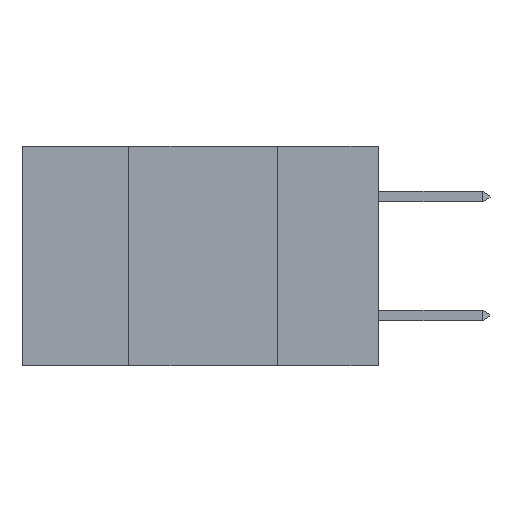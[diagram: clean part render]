
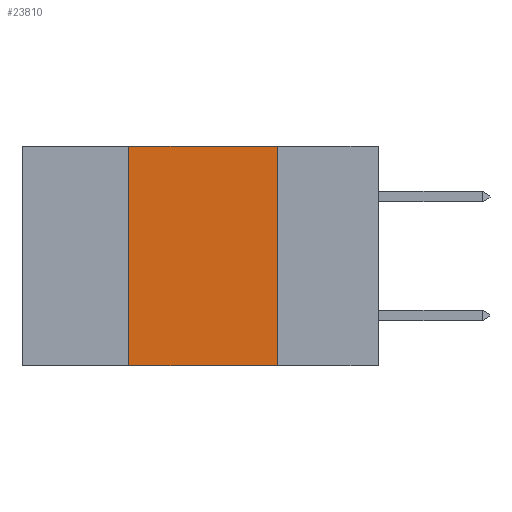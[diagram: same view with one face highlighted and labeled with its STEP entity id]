
A CAD part, left-side view. The second image highlights one B-rep face of the part: STEP entity #23810.
In plain terms, the highlighted planar face has unit normal (-1, 0, 0).
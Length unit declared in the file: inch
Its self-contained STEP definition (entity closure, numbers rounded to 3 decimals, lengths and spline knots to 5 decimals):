
#180 = DIRECTION ( 'NONE',  ( 0., 0., 1. ) ) ;
#444 = ORIENTED_EDGE ( 'NONE', *, *, #26952, .F. ) ;
#778 = VECTOR ( 'NONE', #26306, 39.37008 ) ;
#2094 = FACE_OUTER_BOUND ( 'NONE', #16091, .T. ) ;
#2271 = CARTESIAN_POINT ( 'NONE',  ( 0., 0.42, -0.37 ) ) ;
#2876 = VECTOR ( 'NONE', #19764, 39.37008 ) ;
#3628 = AXIS2_PLACEMENT_3D ( 'NONE', #6539, #8759, #23642 ) ;
#4465 = PLANE ( 'NONE',  #3628 ) ;
#6539 = CARTESIAN_POINT ( 'NONE',  ( 0., 0.6, 0. ) ) ;
#7000 = CARTESIAN_POINT ( 'NONE',  ( 0., 0.6, -0.37 ) ) ;
#8008 = LINE ( 'NONE', #15109, #14369 ) ;
#8246 = EDGE_CURVE ( 'NONE', #8930, #19186, #8008, .T. ) ;
#8759 = DIRECTION ( 'NONE',  ( 1., 0., 0. ) ) ;
#8930 = VERTEX_POINT ( 'NONE', #2271 ) ;
#9194 = CARTESIAN_POINT ( 'NONE',  ( 0., 0.17, 0. ) ) ;
#10628 = CARTESIAN_POINT ( 'NONE',  ( 0., 0.17, -0.37 ) ) ;
#12125 = LINE ( 'NONE', #9194, #778 ) ;
#12238 = VERTEX_POINT ( 'NONE', #18319 ) ;
#12837 = CARTESIAN_POINT ( 'NONE',  ( 0., 0.6, 0. ) ) ;
#14369 = VECTOR ( 'NONE', #180, 39.37008 ) ;
#14972 = VERTEX_POINT ( 'NONE', #10628 ) ;
#15109 = CARTESIAN_POINT ( 'NONE',  ( 0., 0.42, 0. ) ) ;
#16091 = EDGE_LOOP ( 'NONE', ( #21774, #444, #17484, #18148 ) ) ;
#16603 = LINE ( 'NONE', #12837, #22865 ) ;
#17484 = ORIENTED_EDGE ( 'NONE', *, *, #8246, .F. ) ;
#18148 = ORIENTED_EDGE ( 'NONE', *, *, #26421, .T. ) ;
#18319 = CARTESIAN_POINT ( 'NONE',  ( 0., 0.17, 0. ) ) ;
#19186 = VERTEX_POINT ( 'NONE', #20346 ) ;
#19764 = DIRECTION ( 'NONE',  ( 0., -1., 0. ) ) ;
#20346 = CARTESIAN_POINT ( 'NONE',  ( 0., 0.42, 0. ) ) ;
#21502 = DIRECTION ( 'NONE',  ( 0., -1., 0. ) ) ;
#21774 = ORIENTED_EDGE ( 'NONE', *, *, #22697, .F. ) ;
#22697 = EDGE_CURVE ( 'NONE', #12238, #14972, #12125, .T. ) ;
#22865 = VECTOR ( 'NONE', #21502, 39.37008 ) ;
#23642 = DIRECTION ( 'NONE',  ( 0., 0., -1. ) ) ;
#23810 = ADVANCED_FACE ( 'NONE', ( #2094 ), #4465, .F. ) ;
#26306 = DIRECTION ( 'NONE',  ( 0., 0., -1. ) ) ;
#26421 = EDGE_CURVE ( 'NONE', #8930, #14972, #26893, .T. ) ;
#26893 = LINE ( 'NONE', #7000, #2876 ) ;
#26952 = EDGE_CURVE ( 'NONE', #19186, #12238, #16603, .T. ) ;
